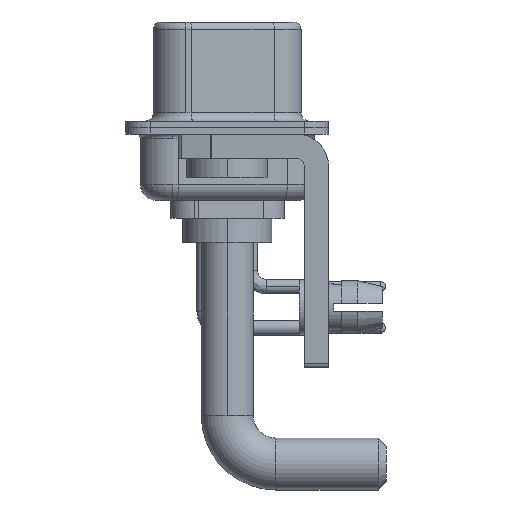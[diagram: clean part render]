
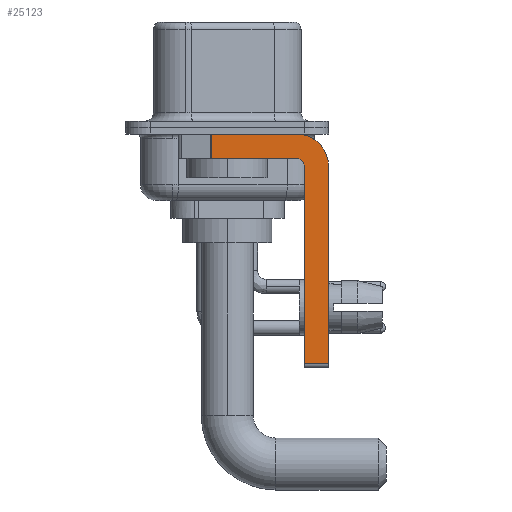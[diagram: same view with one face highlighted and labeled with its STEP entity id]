
A CAD part, left-side view. The second image highlights one B-rep face of the part: STEP entity #25123.
In plain terms, the highlighted planar face has unit normal (-1, 0, 0).
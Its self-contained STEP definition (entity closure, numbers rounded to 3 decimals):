
#159 = CARTESIAN_POINT ( 'NONE',  ( -2.9, -4.25, -2.4 ) ) ;
#463 = VERTEX_POINT ( 'NONE', #20831 ) ;
#568 = DIRECTION ( 'NONE',  ( 0., 0., -1. ) ) ;
#612 = ORIENTED_EDGE ( 'NONE', *, *, #689, .F. ) ;
#689 = EDGE_CURVE ( 'NONE', #2817, #463, #13268, .T. ) ;
#862 = VECTOR ( 'NONE', #11778, 1000. ) ;
#1048 = ORIENTED_EDGE ( 'NONE', *, *, #4699, .F. ) ;
#1549 = DIRECTION ( 'NONE',  ( -1., 0., 0. ) ) ;
#1676 = CARTESIAN_POINT ( 'NONE',  ( -2.9, -4.25, -2.4 ) ) ;
#1762 = VERTEX_POINT ( 'NONE', #15819 ) ;
#2688 = PLANE ( 'NONE',  #14601 ) ;
#2817 = VERTEX_POINT ( 'NONE', #7395 ) ;
#3015 = LINE ( 'NONE', #11087, #9964 ) ;
#3224 = AXIS2_PLACEMENT_3D ( 'NONE', #159, #24657, #20159 ) ;
#4124 = CARTESIAN_POINT ( 'NONE',  ( -2.9, -4.25, -14.55 ) ) ;
#4422 = EDGE_CURVE ( 'NONE', #5500, #2817, #14661, .T. ) ;
#4699 = EDGE_CURVE ( 'NONE', #1762, #5500, #17826, .T. ) ;
#5291 = ORIENTED_EDGE ( 'NONE', *, *, #6366, .F. ) ;
#5500 = VERTEX_POINT ( 'NONE', #6240 ) ;
#6091 = CARTESIAN_POINT ( 'NONE',  ( -2.9, 0.978, -1.9 ) ) ;
#6215 = VECTOR ( 'NONE', #18221, 1000. ) ;
#6240 = CARTESIAN_POINT ( 'NONE',  ( -2.9, -4.25, -0.4 ) ) ;
#6366 = EDGE_CURVE ( 'NONE', #10715, #24504, #10506, .T. ) ;
#6540 = ORIENTED_EDGE ( 'NONE', *, *, #13844, .T. ) ;
#6910 = DIRECTION ( 'NONE',  ( 0., 0., -1. ) ) ;
#7395 = CARTESIAN_POINT ( 'NONE',  ( -2.9, -6.25, -2.4 ) ) ;
#8101 = ORIENTED_EDGE ( 'NONE', *, *, #13676, .F. ) ;
#9109 = DIRECTION ( 'NONE',  ( 0., 1., 0. ) ) ;
#9325 = ORIENTED_EDGE ( 'NONE', *, *, #4422, .F. ) ;
#9335 = CARTESIAN_POINT ( 'NONE',  ( -2.9, 0.978, -1.9 ) ) ;
#9666 = LINE ( 'NONE', #6091, #862 ) ;
#9810 = ORIENTED_EDGE ( 'NONE', *, *, #9989, .T. ) ;
#9947 = ORIENTED_EDGE ( 'NONE', *, *, #24308, .F. ) ;
#9964 = VECTOR ( 'NONE', #9109, 1000. ) ;
#9989 = EDGE_CURVE ( 'NONE', #1762, #26027, #9666, .T. ) ;
#10506 = CIRCLE ( 'NONE', #14753, 0.5 ) ;
#10702 = VECTOR ( 'NONE', #22406, 1000. ) ;
#10715 = VERTEX_POINT ( 'NONE', #25090 ) ;
#11087 = CARTESIAN_POINT ( 'NONE',  ( -2.9, -4.25, -1.9 ) ) ;
#11609 = VECTOR ( 'NONE', #6910, 1000. ) ;
#11778 = DIRECTION ( 'NONE',  ( 0., 0., -1. ) ) ;
#12489 = LINE ( 'NONE', #23481, #16669 ) ;
#12717 = CARTESIAN_POINT ( 'NONE',  ( -2.9, -4.75, -14.55 ) ) ;
#13268 = LINE ( 'NONE', #19359, #11609 ) ;
#13676 = EDGE_CURVE ( 'NONE', #14004, #10715, #12489, .T. ) ;
#13844 = EDGE_CURVE ( 'NONE', #14004, #463, #25970, .T. ) ;
#14004 = VERTEX_POINT ( 'NONE', #12717 ) ;
#14601 = AXIS2_PLACEMENT_3D ( 'NONE', #24689, #20702, #568 ) ;
#14661 = CIRCLE ( 'NONE', #3224, 2. ) ;
#14753 = AXIS2_PLACEMENT_3D ( 'NONE', #1676, #1549, #18093 ) ;
#15819 = CARTESIAN_POINT ( 'NONE',  ( -2.9, 0.978, -0.4 ) ) ;
#16117 = CARTESIAN_POINT ( 'NONE',  ( -2.9, 3., -0.4 ) ) ;
#16601 = FACE_OUTER_BOUND ( 'NONE', #21951, .T. ) ;
#16669 = VECTOR ( 'NONE', #21236, 1000. ) ;
#17826 = LINE ( 'NONE', #16117, #6215 ) ;
#18093 = DIRECTION ( 'NONE',  ( 0., 0., 1. ) ) ;
#18221 = DIRECTION ( 'NONE',  ( 0., -1., 0. ) ) ;
#19359 = CARTESIAN_POINT ( 'NONE',  ( -2.9, -6.25, -2.4 ) ) ;
#20159 = DIRECTION ( 'NONE',  ( 0., 0., -1. ) ) ;
#20702 = DIRECTION ( 'NONE',  ( 1., 0., 0. ) ) ;
#20831 = CARTESIAN_POINT ( 'NONE',  ( -2.9, -6.25, -14.55 ) ) ;
#21236 = DIRECTION ( 'NONE',  ( 0., 0., 1. ) ) ;
#21951 = EDGE_LOOP ( 'NONE', ( #1048, #9810, #9947, #5291, #8101, #6540, #612, #9325 ) ) ;
#21956 = CARTESIAN_POINT ( 'NONE',  ( -2.9, -4.25, -1.9 ) ) ;
#22406 = DIRECTION ( 'NONE',  ( 0., -1., 0. ) ) ;
#23481 = CARTESIAN_POINT ( 'NONE',  ( -2.9, -4.75, -14.8 ) ) ;
#24308 = EDGE_CURVE ( 'NONE', #24504, #26027, #3015, .T. ) ;
#24504 = VERTEX_POINT ( 'NONE', #21956 ) ;
#24657 = DIRECTION ( 'NONE',  ( 1., 0., 0. ) ) ;
#24689 = CARTESIAN_POINT ( 'NONE',  ( -2.9, -4.25, -2.4 ) ) ;
#25090 = CARTESIAN_POINT ( 'NONE',  ( -2.9, -4.75, -2.4 ) ) ;
#25123 = ADVANCED_FACE ( 'NONE', ( #16601 ), #2688, .F. ) ;
#25970 = LINE ( 'NONE', #4124, #10702 ) ;
#26027 = VERTEX_POINT ( 'NONE', #9335 ) ;
